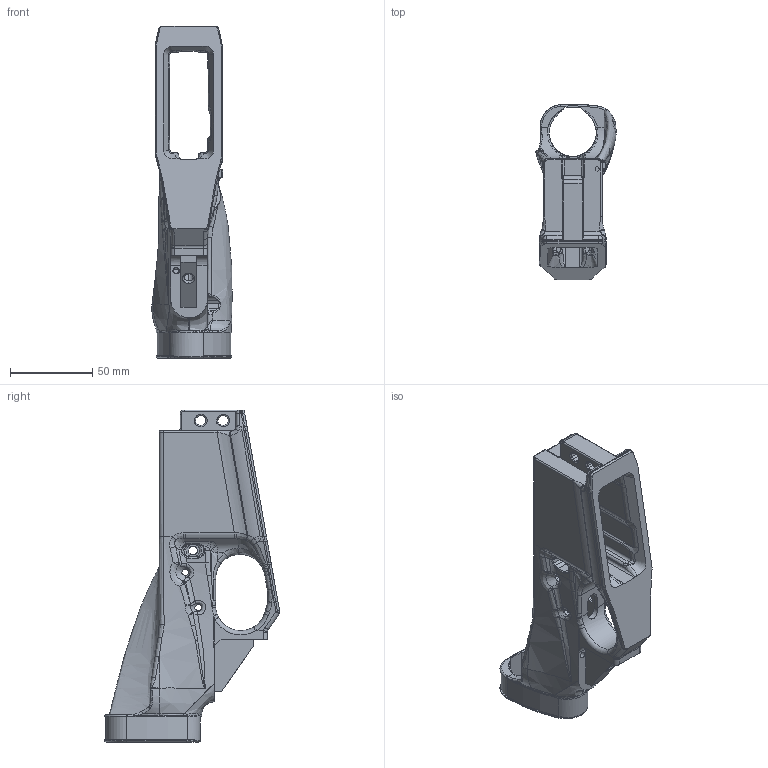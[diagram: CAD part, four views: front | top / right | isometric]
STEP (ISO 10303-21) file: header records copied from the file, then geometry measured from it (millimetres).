
FILE_DESCRIPTION (( 'STEP AP203' ), '1' );
FILE_NAME ('Basic AR-15 Lower V3.0.STEP', '2021-11-11T22:55:43', ( '' ), ( '' ), 'SwSTEP 2.0', 'SolidWorks 2021', '' );
FILE_SCHEMA (( 'CONFIG_CONTROL_DESIGN' ));
Products named in the file (1): Basic AR-15 Lower V3.0
Bounding box: 48.78 x 106.75 x 201.55 mm (x, y, z)
Volume: 178544.3 mm3; surface area: 64784.5 mm2
Topology: 1 solids, 1 shells, 1701 faces, 4473 edges, 2791 vertices
Faces by surface type: bspline 718, plane 533, cylinder 317, torus 88, cone 30, sphere 15
Entity records: 108497 total; most frequent: CARTESIAN_POINT 72488, ORIENTED_EDGE 8866, DIRECTION 5424, EDGE_CURVE 4433, VERTEX_POINT 2791, VECTOR 1816, LINE 1816, AXIS2_PLACEMENT_3D 1804
